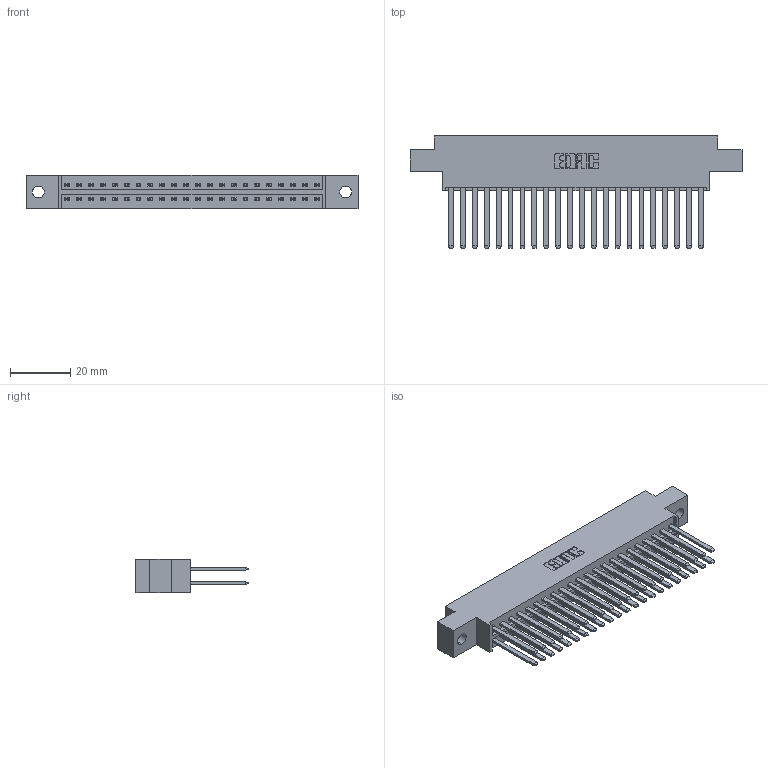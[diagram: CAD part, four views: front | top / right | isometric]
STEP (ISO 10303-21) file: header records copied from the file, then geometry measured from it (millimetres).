
FILE_DESCRIPTION (( 'STEP AP203' ), '1' );
FILE_NAME ('336-044-541-804.STEP', '2020-08-07T23:51:39', ( '' ), ( '' ), 'SwSTEP 2.0', 'SolidWorks 2020', '' );
FILE_SCHEMA (( 'CONFIG_CONTROL_DESIGN' ));
Length unit declared in the file: inch
Products named in the file (3): 336-044-541-804; 336 Part_Offset - .156 Dia - TH; 336-290-001_336-290-541
Assembly tree (45 placements, depth 2):
  336-044-541-804
    336 Part_Offset - .156 Dia - TH
    336-290-001_336-290-541  x44
Bounding box: 110.57 x 37.34 x 11.1 mm (x, y, z)
Volume: 16335.3 mm3; surface area: 20373.9 mm2
Topology: 45 solids, 45 shells, 1966 faces, 5911 edges, 3910 vertices
Faces by surface type: plane 1218, cylinder 748
Entity records: 19498 total; most frequent: CARTESIAN_POINT 3385, ORIENTED_EDGE 3222, DIRECTION 2819, EDGE_CURVE 1611, LINE 1479, VECTOR 1479, VERTEX_POINT 1072, AXIS2_PLACEMENT_3D 670
